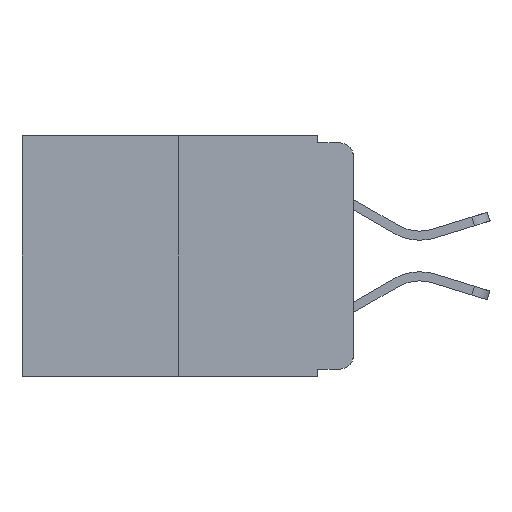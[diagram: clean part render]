
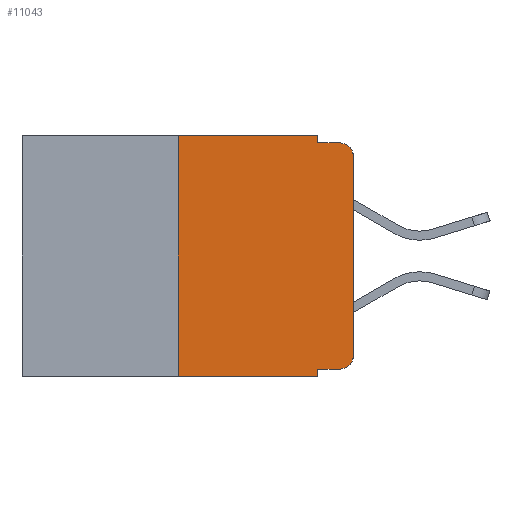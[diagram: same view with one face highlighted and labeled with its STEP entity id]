
A CAD part, left-side view. The second image highlights one B-rep face of the part: STEP entity #11043.
In plain terms, the highlighted planar face has unit normal (-1, 0, 0).
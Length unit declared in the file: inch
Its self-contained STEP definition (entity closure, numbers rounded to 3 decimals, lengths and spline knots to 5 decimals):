
#338 = DIRECTION ( 'NONE',  ( 0., -1., 0. ) ) ;
#610 = VERTEX_POINT ( 'NONE', #9327 ) ;
#837 = ORIENTED_EDGE ( 'NONE', *, *, #1773, .T. ) ;
#922 = VERTEX_POINT ( 'NONE', #7123 ) ;
#1095 = DIRECTION ( 'NONE',  ( 0., -1., 0. ) ) ;
#1180 = DIRECTION ( 'NONE',  ( 0., -1., 0. ) ) ;
#1290 = EDGE_CURVE ( 'NONE', #610, #9083, #7189, .T. ) ;
#1459 = PLANE ( 'NONE',  #1915 ) ;
#1725 = CARTESIAN_POINT ( 'NONE',  ( 0., 0.473, 0. ) ) ;
#1773 = EDGE_CURVE ( 'NONE', #9059, #922, #20510, .T. ) ;
#1915 = AXIS2_PLACEMENT_3D ( 'NONE', #1725, #7306, #17235 ) ;
#2437 = LINE ( 'NONE', #10198, #13637 ) ;
#2689 = AXIS2_PLACEMENT_3D ( 'NONE', #22373, #10191, #24188 ) ;
#2797 = CARTESIAN_POINT ( 'NONE',  ( 0., 0.051, -0.343 ) ) ;
#2980 = DIRECTION ( 'NONE',  ( 0., 0., -1. ) ) ;
#3409 = EDGE_CURVE ( 'NONE', #22247, #610, #13971, .T. ) ;
#3716 = EDGE_CURVE ( 'NONE', #9059, #17580, #15110, .T. ) ;
#3899 = DIRECTION ( 'NONE',  ( 0., 0., -1. ) ) ;
#4388 = ORIENTED_EDGE ( 'NONE', *, *, #3409, .F. ) ;
#4453 = ORIENTED_EDGE ( 'NONE', *, *, #13760, .T. ) ;
#4512 = ORIENTED_EDGE ( 'NONE', *, *, #6925, .F. ) ;
#4878 = EDGE_CURVE ( 'NONE', #22247, #17580, #10125, .T. ) ;
#5247 = CARTESIAN_POINT ( 'NONE',  ( 0., 0.473, 0. ) ) ;
#5418 = EDGE_LOOP ( 'NONE', ( #4453, #21223, #21894, #4512, #19075, #4388, #22437, #15093, #837, #10675 ) ) ;
#5760 = VECTOR ( 'NONE', #16062, 39.37008 ) ;
#5911 = VECTOR ( 'NONE', #11521, 39.37008 ) ;
#6375 = DIRECTION ( 'NONE',  ( 0., 0., 1. ) ) ;
#6925 = EDGE_CURVE ( 'NONE', #9083, #24224, #12780, .T. ) ;
#7123 = CARTESIAN_POINT ( 'NONE',  ( 0., 0.02, -0.333 ) ) ;
#7189 = LINE ( 'NONE', #5247, #21514 ) ;
#7306 = DIRECTION ( 'NONE',  ( 1., 0., 0. ) ) ;
#7506 = DIRECTION ( 'NONE',  ( -1., 0., 0. ) ) ;
#8755 = CARTESIAN_POINT ( 'NONE',  ( 0., 0.25, -0.343 ) ) ;
#8999 = EDGE_CURVE ( 'NONE', #23410, #21104, #23766, .T. ) ;
#9059 = VERTEX_POINT ( 'NONE', #12126 ) ;
#9083 = VERTEX_POINT ( 'NONE', #23919 ) ;
#9310 = CARTESIAN_POINT ( 'NONE',  ( 0., 0.051, 0. ) ) ;
#9327 = CARTESIAN_POINT ( 'NONE',  ( 0., 0.25, 0. ) ) ;
#9864 = FACE_OUTER_BOUND ( 'NONE', #5418, .T. ) ;
#10125 = LINE ( 'NONE', #11794, #5911 ) ;
#10191 = DIRECTION ( 'NONE',  ( -1., 0., 0. ) ) ;
#10198 = CARTESIAN_POINT ( 'NONE',  ( 0., 0.051, -0.01 ) ) ;
#10675 = ORIENTED_EDGE ( 'NONE', *, *, #23192, .T. ) ;
#11043 = ADVANCED_FACE ( 'NONE', ( #9864 ), #1459, .F. ) ;
#11310 = VECTOR ( 'NONE', #3899, 39.37008 ) ;
#11521 = DIRECTION ( 'NONE',  ( 0., -1., 0. ) ) ;
#11794 = CARTESIAN_POINT ( 'NONE',  ( 0., 0.473, -0.343 ) ) ;
#12034 = VECTOR ( 'NONE', #2980, 39.37008 ) ;
#12126 = CARTESIAN_POINT ( 'NONE',  ( 0., 0.051, -0.333 ) ) ;
#12780 = LINE ( 'NONE', #23011, #12034 ) ;
#12813 = CIRCLE ( 'NONE', #21981, 0.02 ) ;
#13637 = VECTOR ( 'NONE', #338, 39.37008 ) ;
#13760 = EDGE_CURVE ( 'NONE', #24164, #23410, #13975, .T. ) ;
#13971 = LINE ( 'NONE', #18247, #17510 ) ;
#13975 = LINE ( 'NONE', #20221, #5760 ) ;
#15093 = ORIENTED_EDGE ( 'NONE', *, *, #3716, .F. ) ;
#15110 = LINE ( 'NONE', #9310, #11310 ) ;
#16062 = DIRECTION ( 'NONE',  ( 0., 0., 1. ) ) ;
#17235 = DIRECTION ( 'NONE',  ( 0., 0., -1. ) ) ;
#17510 = VECTOR ( 'NONE', #6375, 39.37008 ) ;
#17561 = CARTESIAN_POINT ( 'NONE',  ( 0., 0.02, -0.313 ) ) ;
#17580 = VERTEX_POINT ( 'NONE', #2797 ) ;
#17747 = VECTOR ( 'NONE', #1180, 39.37008 ) ;
#18247 = CARTESIAN_POINT ( 'NONE',  ( 0., 0.25, 0. ) ) ;
#18786 = CARTESIAN_POINT ( 'NONE',  ( 0., 0.051, -0.333 ) ) ;
#19075 = ORIENTED_EDGE ( 'NONE', *, *, #1290, .F. ) ;
#19973 = CARTESIAN_POINT ( 'NONE',  ( 0., 0.02, -0.01 ) ) ;
#20221 = CARTESIAN_POINT ( 'NONE',  ( 0., 0., 0. ) ) ;
#20510 = LINE ( 'NONE', #18786, #17747 ) ;
#21104 = VERTEX_POINT ( 'NONE', #19973 ) ;
#21223 = ORIENTED_EDGE ( 'NONE', *, *, #8999, .T. ) ;
#21514 = VECTOR ( 'NONE', #1095, 39.37008 ) ;
#21894 = ORIENTED_EDGE ( 'NONE', *, *, #24677, .F. ) ;
#21981 = AXIS2_PLACEMENT_3D ( 'NONE', #17561, #7506, #25506 ) ;
#22016 = CARTESIAN_POINT ( 'NONE',  ( 0., 0., -0.03 ) ) ;
#22247 = VERTEX_POINT ( 'NONE', #8755 ) ;
#22373 = CARTESIAN_POINT ( 'NONE',  ( 0., 0.02, -0.03 ) ) ;
#22437 = ORIENTED_EDGE ( 'NONE', *, *, #4878, .T. ) ;
#23011 = CARTESIAN_POINT ( 'NONE',  ( 0., 0.051, 0. ) ) ;
#23192 = EDGE_CURVE ( 'NONE', #922, #24164, #12813, .T. ) ;
#23410 = VERTEX_POINT ( 'NONE', #22016 ) ;
#23766 = CIRCLE ( 'NONE', #2689, 0.02 ) ;
#23919 = CARTESIAN_POINT ( 'NONE',  ( 0., 0.051, 0. ) ) ;
#24003 = CARTESIAN_POINT ( 'NONE',  ( 0., 0.051, -0.01 ) ) ;
#24164 = VERTEX_POINT ( 'NONE', #25175 ) ;
#24188 = DIRECTION ( 'NONE',  ( 0., 0., -1. ) ) ;
#24224 = VERTEX_POINT ( 'NONE', #24003 ) ;
#24677 = EDGE_CURVE ( 'NONE', #24224, #21104, #2437, .T. ) ;
#25175 = CARTESIAN_POINT ( 'NONE',  ( 0., 0., -0.313 ) ) ;
#25506 = DIRECTION ( 'NONE',  ( 0., 0., -1. ) ) ;
